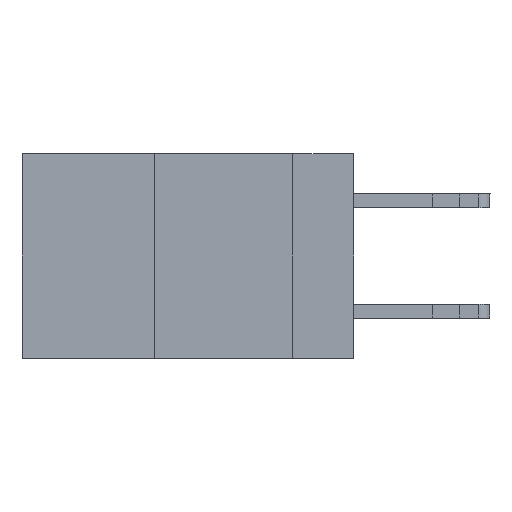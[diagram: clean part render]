
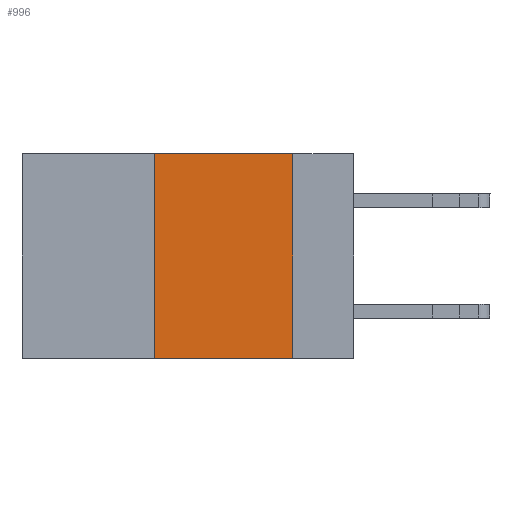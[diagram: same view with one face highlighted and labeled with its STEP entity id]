
A CAD part, left-side view. The second image highlights one B-rep face of the part: STEP entity #996.
In plain terms, the highlighted planar face has unit normal (-1, 0, 0).
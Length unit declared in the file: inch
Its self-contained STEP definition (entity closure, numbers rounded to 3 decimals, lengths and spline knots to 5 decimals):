
#471 = ORIENTED_EDGE ( 'NONE', *, *, #11840, .T. ) ;
#996 = ADVANCED_FACE ( 'NONE', ( #7686 ), #6130, .F. ) ;
#1540 = ORIENTED_EDGE ( 'NONE', *, *, #21053, .F. ) ;
#2239 = VECTOR ( 'NONE', #21747, 39.37008 ) ;
#2306 = CARTESIAN_POINT ( 'NONE',  ( 0., 0.36, 0. ) ) ;
#3316 = EDGE_CURVE ( 'NONE', #14855, #8814, #11663, .T. ) ;
#3832 = CARTESIAN_POINT ( 'NONE',  ( 0., 0.6, 0. ) ) ;
#6130 = PLANE ( 'NONE',  #14733 ) ;
#6518 = CARTESIAN_POINT ( 'NONE',  ( 0., 0.6, 0. ) ) ;
#7099 = ORIENTED_EDGE ( 'NONE', *, *, #12303, .F. ) ;
#7454 = LINE ( 'NONE', #3832, #20148 ) ;
#7474 = LINE ( 'NONE', #7987, #2239 ) ;
#7686 = FACE_OUTER_BOUND ( 'NONE', #19330, .T. ) ;
#7987 = CARTESIAN_POINT ( 'NONE',  ( 0., 0.6, -0.37 ) ) ;
#8814 = VERTEX_POINT ( 'NONE', #2306 ) ;
#9626 = CARTESIAN_POINT ( 'NONE',  ( 0., 0.36, -0.37 ) ) ;
#9782 = VECTOR ( 'NONE', #21691, 39.37008 ) ;
#10228 = CARTESIAN_POINT ( 'NONE',  ( 0., 0.11, -0.37 ) ) ;
#10588 = VECTOR ( 'NONE', #20141, 39.37008 ) ;
#11087 = DIRECTION ( 'NONE',  ( 0., 0., -1. ) ) ;
#11585 = DIRECTION ( 'NONE',  ( 1., 0., 0. ) ) ;
#11663 = LINE ( 'NONE', #18379, #10588 ) ;
#11840 = EDGE_CURVE ( 'NONE', #14855, #22349, #7474, .T. ) ;
#12303 = EDGE_CURVE ( 'NONE', #8814, #15582, #7454, .T. ) ;
#12650 = DIRECTION ( 'NONE',  ( 0., -1., 0. ) ) ;
#14733 = AXIS2_PLACEMENT_3D ( 'NONE', #6518, #11585, #11087 ) ;
#14855 = VERTEX_POINT ( 'NONE', #9626 ) ;
#15582 = VERTEX_POINT ( 'NONE', #21901 ) ;
#18346 = ORIENTED_EDGE ( 'NONE', *, *, #3316, .F. ) ;
#18379 = CARTESIAN_POINT ( 'NONE',  ( 0., 0.36, 0. ) ) ;
#19330 = EDGE_LOOP ( 'NONE', ( #1540, #7099, #18346, #471 ) ) ;
#19412 = LINE ( 'NONE', #19968, #9782 ) ;
#19968 = CARTESIAN_POINT ( 'NONE',  ( 0., 0.11, 0. ) ) ;
#20141 = DIRECTION ( 'NONE',  ( 0., 0., 1. ) ) ;
#20148 = VECTOR ( 'NONE', #12650, 39.37008 ) ;
#21053 = EDGE_CURVE ( 'NONE', #15582, #22349, #19412, .T. ) ;
#21691 = DIRECTION ( 'NONE',  ( 0., 0., -1. ) ) ;
#21747 = DIRECTION ( 'NONE',  ( 0., -1., 0. ) ) ;
#21901 = CARTESIAN_POINT ( 'NONE',  ( 0., 0.11, 0. ) ) ;
#22349 = VERTEX_POINT ( 'NONE', #10228 ) ;
